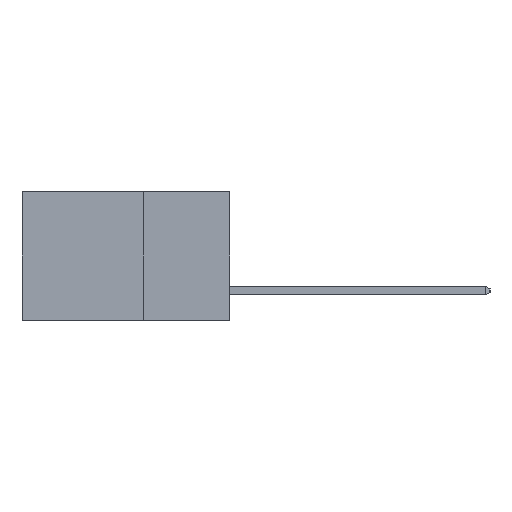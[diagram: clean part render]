
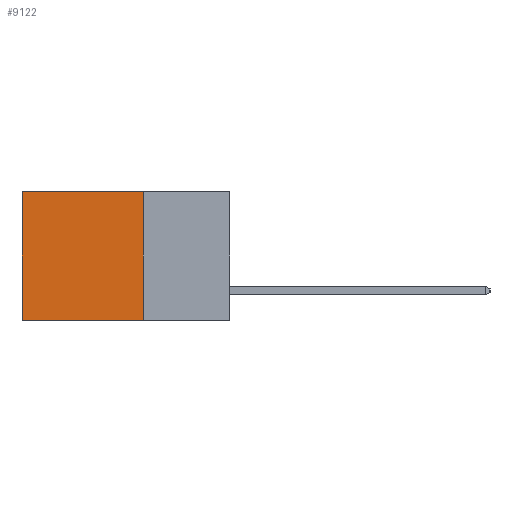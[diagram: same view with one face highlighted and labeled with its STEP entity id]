
A CAD part, left-side view. The second image highlights one B-rep face of the part: STEP entity #9122.
In plain terms, the highlighted planar face has unit normal (-1, 0, 0).
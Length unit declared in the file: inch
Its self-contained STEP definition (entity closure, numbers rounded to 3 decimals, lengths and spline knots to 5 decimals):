
#120 = VECTOR ( 'NONE', #10837, 39.37008 ) ;
#450 = EDGE_CURVE ( 'NONE', #6867, #10122, #1974, .T. ) ;
#458 = DIRECTION ( 'NONE',  ( 0., 1., 0. ) ) ;
#608 = FACE_OUTER_BOUND ( 'NONE', #4711, .T. ) ;
#1030 = CARTESIAN_POINT ( 'NONE',  ( 0.298, 0.25, 0. ) ) ;
#1379 = VECTOR ( 'NONE', #6736, 39.37008 ) ;
#1974 = LINE ( 'NONE', #1030, #13367 ) ;
#3394 = DIRECTION ( 'NONE',  ( 1., 0., 0. ) ) ;
#3706 = LINE ( 'NONE', #12026, #120 ) ;
#3719 = CARTESIAN_POINT ( 'NONE',  ( 0.298, 0.25, -0.37 ) ) ;
#3940 = ORIENTED_EDGE ( 'NONE', *, *, #12810, .F. ) ;
#4313 = CARTESIAN_POINT ( 'NONE',  ( 0.298, 0.6, 0. ) ) ;
#4552 = LINE ( 'NONE', #4313, #1379 ) ;
#4711 = EDGE_LOOP ( 'NONE', ( #14461, #5007, #3940, #10502 ) ) ;
#4761 = EDGE_CURVE ( 'NONE', #8554, #12847, #11614, .T. ) ;
#5007 = ORIENTED_EDGE ( 'NONE', *, *, #4761, .F. ) ;
#5193 = CARTESIAN_POINT ( 'NONE',  ( 0.298, 0.25, 0. ) ) ;
#6736 = DIRECTION ( 'NONE',  ( 0., 0., -1. ) ) ;
#6867 = VERTEX_POINT ( 'NONE', #5193 ) ;
#6926 = AXIS2_PLACEMENT_3D ( 'NONE', #15055, #3394, #11617 ) ;
#7686 = CARTESIAN_POINT ( 'NONE',  ( 0.298, 0.25, -0.37 ) ) ;
#7695 = CARTESIAN_POINT ( 'NONE',  ( 0.298, 0.6, 0. ) ) ;
#8554 = VERTEX_POINT ( 'NONE', #3719 ) ;
#9122 = ADVANCED_FACE ( 'NONE', ( #608 ), #10449, .F. ) ;
#10122 = VERTEX_POINT ( 'NONE', #7695 ) ;
#10449 = PLANE ( 'NONE',  #6926 ) ;
#10502 = ORIENTED_EDGE ( 'NONE', *, *, #450, .T. ) ;
#10837 = DIRECTION ( 'NONE',  ( 0., 0., -1. ) ) ;
#10933 = CARTESIAN_POINT ( 'NONE',  ( 0.298, 0.6, -0.37 ) ) ;
#11614 = LINE ( 'NONE', #7686, #14307 ) ;
#11617 = DIRECTION ( 'NONE',  ( 0., 0., -1. ) ) ;
#12026 = CARTESIAN_POINT ( 'NONE',  ( 0.298, 0.25, 0. ) ) ;
#12810 = EDGE_CURVE ( 'NONE', #6867, #8554, #3706, .T. ) ;
#12847 = VERTEX_POINT ( 'NONE', #10933 ) ;
#13367 = VECTOR ( 'NONE', #458, 39.37008 ) ;
#14307 = VECTOR ( 'NONE', #14664, 39.37008 ) ;
#14461 = ORIENTED_EDGE ( 'NONE', *, *, #14633, .T. ) ;
#14633 = EDGE_CURVE ( 'NONE', #10122, #12847, #4552, .T. ) ;
#14664 = DIRECTION ( 'NONE',  ( 0., 1., 0. ) ) ;
#15055 = CARTESIAN_POINT ( 'NONE',  ( 0.298, 0.25, 0. ) ) ;
